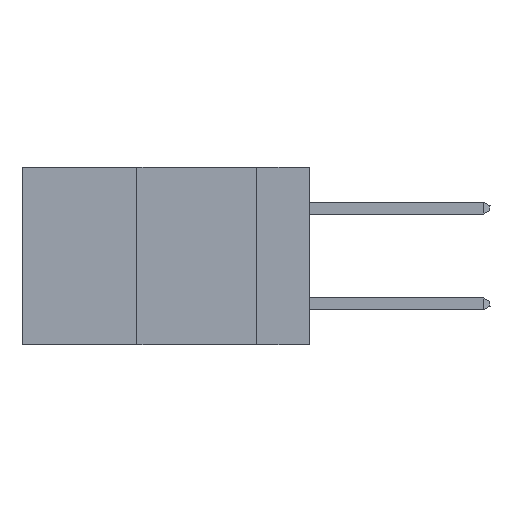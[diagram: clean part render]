
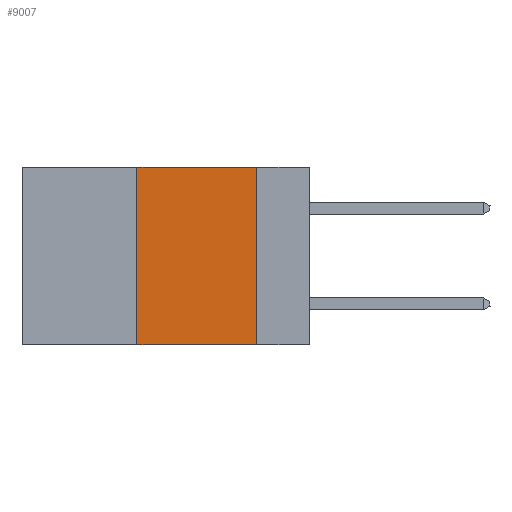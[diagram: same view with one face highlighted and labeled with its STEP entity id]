
A CAD part, left-side view. The second image highlights one B-rep face of the part: STEP entity #9007.
In plain terms, the highlighted planar face has unit normal (-1, 0, 0).
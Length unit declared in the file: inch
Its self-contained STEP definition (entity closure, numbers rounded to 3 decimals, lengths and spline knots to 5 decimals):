
#195 = CARTESIAN_POINT ( 'NONE',  ( 0., 0.36, 0. ) ) ;
#220 = FACE_OUTER_BOUND ( 'NONE', #13343, .T. ) ;
#766 = VECTOR ( 'NONE', #12137, 39.37008 ) ;
#825 = CARTESIAN_POINT ( 'NONE',  ( 0., 0.11, 0. ) ) ;
#887 = CARTESIAN_POINT ( 'NONE',  ( 0., 0.11, 0. ) ) ;
#1222 = DIRECTION ( 'NONE',  ( 0., 0., -1. ) ) ;
#2562 = EDGE_CURVE ( 'NONE', #12154, #7239, #15155, .T. ) ;
#3507 = LINE ( 'NONE', #15513, #14046 ) ;
#3541 = LINE ( 'NONE', #13512, #766 ) ;
#3701 = CARTESIAN_POINT ( 'NONE',  ( 0., 0.36, -0.37 ) ) ;
#3807 = ORIENTED_EDGE ( 'NONE', *, *, #2562, .F. ) ;
#5461 = CARTESIAN_POINT ( 'NONE',  ( 0., 0.6, -0.37 ) ) ;
#6049 = ORIENTED_EDGE ( 'NONE', *, *, #8350, .F. ) ;
#6643 = CARTESIAN_POINT ( 'NONE',  ( 0., 0.11, -0.37 ) ) ;
#6969 = PLANE ( 'NONE',  #11372 ) ;
#7239 = VERTEX_POINT ( 'NONE', #6643 ) ;
#7580 = EDGE_CURVE ( 'NONE', #13659, #12154, #3541, .T. ) ;
#8350 = EDGE_CURVE ( 'NONE', #18247, #13659, #3507, .T. ) ;
#9007 = ADVANCED_FACE ( 'NONE', ( #220 ), #6969, .F. ) ;
#9842 = DIRECTION ( 'NONE',  ( 0., 0., -1. ) ) ;
#10980 = DIRECTION ( 'NONE',  ( 0., 0., 1. ) ) ;
#11372 = AXIS2_PLACEMENT_3D ( 'NONE', #11550, #17430, #1222 ) ;
#11550 = CARTESIAN_POINT ( 'NONE',  ( 0., 0.6, 0. ) ) ;
#12137 = DIRECTION ( 'NONE',  ( 0., -1., 0. ) ) ;
#12154 = VERTEX_POINT ( 'NONE', #887 ) ;
#12409 = ORIENTED_EDGE ( 'NONE', *, *, #7580, .F. ) ;
#12801 = DIRECTION ( 'NONE',  ( 0., -1., 0. ) ) ;
#13343 = EDGE_LOOP ( 'NONE', ( #3807, #12409, #6049, #16142 ) ) ;
#13512 = CARTESIAN_POINT ( 'NONE',  ( 0., 0.6, 0. ) ) ;
#13659 = VERTEX_POINT ( 'NONE', #195 ) ;
#14046 = VECTOR ( 'NONE', #10980, 39.37008 ) ;
#14535 = EDGE_CURVE ( 'NONE', #18247, #7239, #16872, .T. ) ;
#14668 = VECTOR ( 'NONE', #9842, 39.37008 ) ;
#15155 = LINE ( 'NONE', #825, #14668 ) ;
#15513 = CARTESIAN_POINT ( 'NONE',  ( 0., 0.36, 0. ) ) ;
#16142 = ORIENTED_EDGE ( 'NONE', *, *, #14535, .T. ) ;
#16872 = LINE ( 'NONE', #5461, #17114 ) ;
#17114 = VECTOR ( 'NONE', #12801, 39.37008 ) ;
#17430 = DIRECTION ( 'NONE',  ( 1., 0., 0. ) ) ;
#18247 = VERTEX_POINT ( 'NONE', #3701 ) ;
